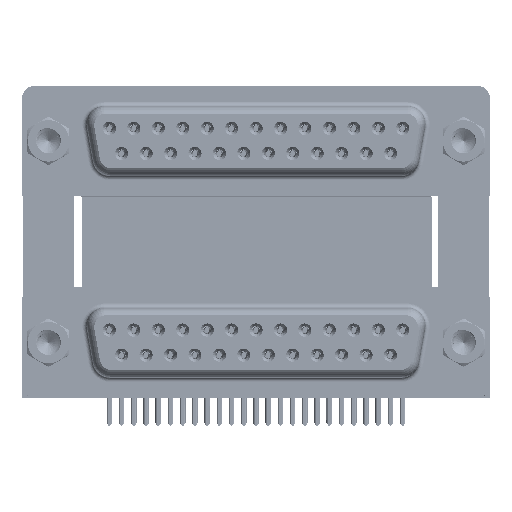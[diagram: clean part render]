
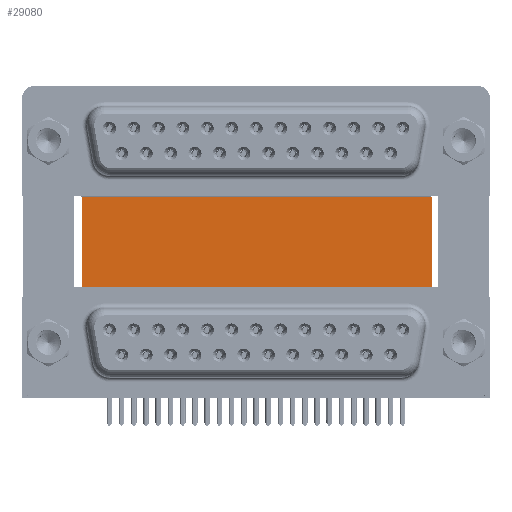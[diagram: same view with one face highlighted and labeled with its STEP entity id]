
A CAD part, top view. The second image highlights one B-rep face of the part: STEP entity #29080.
In plain terms, the highlighted planar face has unit normal (0, 0, 1).
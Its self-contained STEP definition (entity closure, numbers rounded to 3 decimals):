
#541 = EDGE_LOOP ( 'NONE', ( #42336, #49119, #2415, #38428 ) ) ;
#1329 = PLANE ( 'NONE',  #43206 ) ;
#1967 = DIRECTION ( 'NONE',  ( 0., 0., -1. ) ) ;
#2415 = ORIENTED_EDGE ( 'NONE', *, *, #60652, .F. ) ;
#2949 = VECTOR ( 'NONE', #4561, 1000. ) ;
#4443 = DIRECTION ( 'NONE',  ( 1., 0., 0. ) ) ;
#4561 = DIRECTION ( 'NONE',  ( 1., 0., 0. ) ) ;
#6673 = LINE ( 'NONE', #36405, #36573 ) ;
#7642 = VERTEX_POINT ( 'NONE', #25490 ) ;
#9406 = CARTESIAN_POINT ( 'NONE',  ( 3.79, 16.585, -12. ) ) ;
#11228 = LINE ( 'NONE', #36642, #26024 ) ;
#16510 = DIRECTION ( 'NONE',  ( 0., -1., 0. ) ) ;
#17248 = CARTESIAN_POINT ( 'NONE',  ( 43.43, 16.585, -12. ) ) ;
#19655 = VERTEX_POINT ( 'NONE', #17248 ) ;
#21163 = FACE_OUTER_BOUND ( 'NONE', #541, .T. ) ;
#25490 = CARTESIAN_POINT ( 'NONE',  ( 43.43, -3.735, -12. ) ) ;
#26024 = VECTOR ( 'NONE', #16510, 1000. ) ;
#29080 = ADVANCED_FACE ( 'NONE', ( #21163 ), #1329, .F. ) ;
#29656 = CARTESIAN_POINT ( 'NONE',  ( 3.79, -3.735, -12. ) ) ;
#34948 = CARTESIAN_POINT ( 'NONE',  ( 3.79, -3.735, -12. ) ) ;
#36405 = CARTESIAN_POINT ( 'NONE',  ( 3.79, 16.585, -12. ) ) ;
#36573 = VECTOR ( 'NONE', #56195, 1000. ) ;
#36642 = CARTESIAN_POINT ( 'NONE',  ( 43.43, 16.585, -12. ) ) ;
#38428 = ORIENTED_EDGE ( 'NONE', *, *, #62964, .T. ) ;
#42200 = EDGE_CURVE ( 'NONE', #19655, #7642, #11228, .T. ) ;
#42336 = ORIENTED_EDGE ( 'NONE', *, *, #64952, .T. ) ;
#43206 = AXIS2_PLACEMENT_3D ( 'NONE', #57121, #1967, #51519 ) ;
#46907 = VECTOR ( 'NONE', #4443, 1000. ) ;
#49119 = ORIENTED_EDGE ( 'NONE', *, *, #42200, .F. ) ;
#49468 = LINE ( 'NONE', #34948, #2949 ) ;
#50191 = VERTEX_POINT ( 'NONE', #53056 ) ;
#51519 = DIRECTION ( 'NONE',  ( -1., 0., 0. ) ) ;
#53056 = CARTESIAN_POINT ( 'NONE',  ( 3.79, 16.585, -12. ) ) ;
#55920 = LINE ( 'NONE', #9406, #46907 ) ;
#56195 = DIRECTION ( 'NONE',  ( 0., -1., 0. ) ) ;
#57121 = CARTESIAN_POINT ( 'NONE',  ( 3.79, 16.585, -12. ) ) ;
#60652 = EDGE_CURVE ( 'NONE', #50191, #19655, #55920, .T. ) ;
#62964 = EDGE_CURVE ( 'NONE', #50191, #64981, #6673, .T. ) ;
#64952 = EDGE_CURVE ( 'NONE', #64981, #7642, #49468, .T. ) ;
#64981 = VERTEX_POINT ( 'NONE', #29656 ) ;
